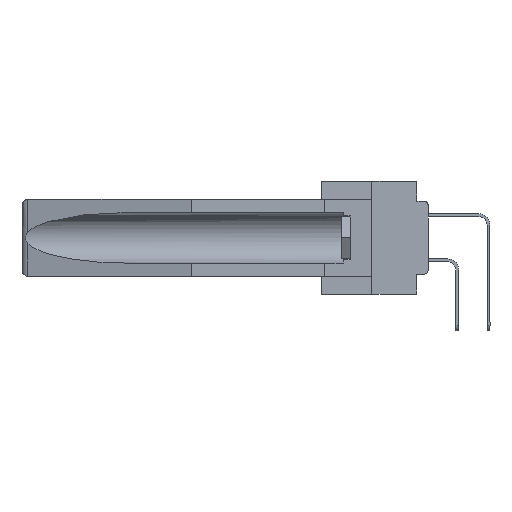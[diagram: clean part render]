
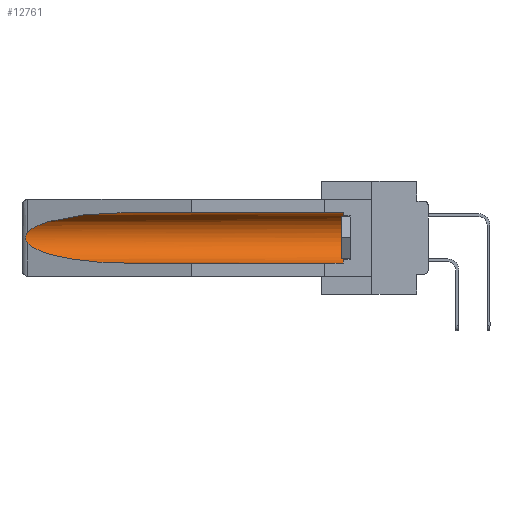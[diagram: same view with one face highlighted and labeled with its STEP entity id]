
A CAD part, left-side view. The second image highlights one B-rep face of the part: STEP entity #12761.
In plain terms, the highlighted cylindrical face has radius 2.857 mm (diameter 5.715 mm), a partial arc.
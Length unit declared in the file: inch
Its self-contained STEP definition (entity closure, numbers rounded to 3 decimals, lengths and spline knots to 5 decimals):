
#741 = DIRECTION ( 'NONE',  ( 0., -1., 0. ) ) ;
#1095 = VERTEX_POINT ( 'NONE', #1734 ) ;
#1589 = CARTESIAN_POINT ( 'NONE',  ( 0.26654, 1.53092, -0.15636 ) ) ;
#1707 =( BOUNDED_CURVE ( )  B_SPLINE_CURVE ( 3, ( #26544, #2659, #31917, #33365 ),
 .UNSPECIFIED., .F., .T. ) 
 B_SPLINE_CURVE_WITH_KNOTS ( ( 4, 4 ),
 ( 0.1948, 1.5708 ),
 .UNSPECIFIED. ) 
 CURVE ( )  GEOMETRIC_REPRESENTATION_ITEM ( )  RATIONAL_B_SPLINE_CURVE ( ( 1., 0.848, 0.848, 1. ) ) 
 REPRESENTATION_ITEM ( '' )  );
#1734 = CARTESIAN_POINT ( 'NONE',  ( 0.155, 0.126, -0.284 ) ) ;
#1753 = CARTESIAN_POINT ( 'NONE',  ( 0.155, 1.07973, -0.059 ) ) ;
#2185 = DIRECTION ( 'NONE',  ( 0., 1., 0. ) ) ;
#2433 = EDGE_CURVE ( 'NONE', #29137, #6163, #12590, .T. ) ;
#2659 = CARTESIAN_POINT ( 'NONE',  ( 0.25451, 1.48313, -0.24835 ) ) ;
#4751 = B_SPLINE_CURVE_WITH_KNOTS ( 'NONE', 3,
 ( #6805, #23032, #1589, #31147, #17606, #23197, #30980, #7320, #12388, #20214 ),
 .UNSPECIFIED., .F., .F.,
 ( 4, 2, 2, 2, 4 ),
 ( 0., 0.00029, 0.00058, 0.00087, 0.00117 ),
 .UNSPECIFIED. ) ;
#4790 = CYLINDRICAL_SURFACE ( 'NONE', #17360, 0.1125 ) ;
#5153 = EDGE_CURVE ( 'NONE', #28629, #29137, #23954, .T. ) ;
#5501 = ORIENTED_EDGE ( 'NONE', *, *, #9242, .T. ) ;
#6163 = VERTEX_POINT ( 'NONE', #24202 ) ;
#6591 = CARTESIAN_POINT ( 'NONE',  ( 0.155, -0.30754, -0.284 ) ) ;
#6805 = CARTESIAN_POINT ( 'NONE',  ( 0.26537, 1.52718, -0.14972 ) ) ;
#7320 = CARTESIAN_POINT ( 'NONE',  ( 0.26655, 1.53094, -0.18657 ) ) ;
#8758 = CARTESIAN_POINT ( 'NONE',  ( 0.26537, 1.52718, -0.19328 ) ) ;
#9242 = EDGE_CURVE ( 'NONE', #1095, #28629, #21501, .T. ) ;
#9428 = CARTESIAN_POINT ( 'NONE',  ( 0.26537, 1.52718, -0.14972 ) ) ;
#10366 = CARTESIAN_POINT ( 'NONE',  ( 0.155, -0.30754, -0.059 ) ) ;
#11535 = EDGE_CURVE ( 'NONE', #18109, #17452, #1707, .T. ) ;
#11882 = CARTESIAN_POINT ( 'NONE',  ( 0.21114, 1.30732, -0.059 ) ) ;
#12384 = CARTESIAN_POINT ( 'NONE',  ( 0.25451, 1.48313, -0.09465 ) ) ;
#12388 = CARTESIAN_POINT ( 'NONE',  ( 0.26597, 1.5296, -0.19026 ) ) ;
#12590 =( BOUNDED_CURVE ( )  B_SPLINE_CURVE ( 3, ( #1753, #11882, #12384, #9428 ),
 .UNSPECIFIED., .F., .T. ) 
 B_SPLINE_CURVE_WITH_KNOTS ( ( 4, 4 ),
 ( 4.71239, 6.08839 ),
 .UNSPECIFIED. ) 
 CURVE ( )  GEOMETRIC_REPRESENTATION_ITEM ( )  RATIONAL_B_SPLINE_CURVE ( ( 1., 0.848, 0.848, 1. ) ) 
 REPRESENTATION_ITEM ( '' )  );
#12638 = CARTESIAN_POINT ( 'NONE',  ( 0.155, 1.07973, -0.284 ) ) ;
#12761 = ADVANCED_FACE ( 'NONE', ( #30919 ), #4790, .F. ) ;
#12999 = DIRECTION ( 'NONE',  ( 0., 0., 1. ) ) ;
#14518 = CARTESIAN_POINT ( 'NONE',  ( 0.155, 0.126, -0.059 ) ) ;
#15182 = ORIENTED_EDGE ( 'NONE', *, *, #26651, .T. ) ;
#17360 = AXIS2_PLACEMENT_3D ( 'NONE', #28176, #2185, #12999 ) ;
#17452 = VERTEX_POINT ( 'NONE', #12638 ) ;
#17564 = DIRECTION ( 'NONE',  ( 0., 1., 0. ) ) ;
#17606 = CARTESIAN_POINT ( 'NONE',  ( 0.2675, 1.53308, -0.16763 ) ) ;
#17778 = ORIENTED_EDGE ( 'NONE', *, *, #32918, .F. ) ;
#18109 = VERTEX_POINT ( 'NONE', #8758 ) ;
#19148 = ORIENTED_EDGE ( 'NONE', *, *, #11535, .T. ) ;
#19695 = DIRECTION ( 'NONE',  ( 0., 0., 1. ) ) ;
#20214 = CARTESIAN_POINT ( 'NONE',  ( 0.26537, 1.52718, -0.19328 ) ) ;
#20800 = DIRECTION ( 'NONE',  ( 0., 1., 0. ) ) ;
#21501 = CIRCLE ( 'NONE', #33087, 0.1125 ) ;
#22136 = CARTESIAN_POINT ( 'NONE',  ( 0.155, 0.126, -0.1715 ) ) ;
#22277 = CARTESIAN_POINT ( 'NONE',  ( 0.155, 1.07973, -0.059 ) ) ;
#23031 = EDGE_LOOP ( 'NONE', ( #29703, #15182, #19148, #17778, #5501, #27229 ) ) ;
#23032 = CARTESIAN_POINT ( 'NONE',  ( 0.26597, 1.52961, -0.15275 ) ) ;
#23197 = CARTESIAN_POINT ( 'NONE',  ( 0.2675, 1.53308, -0.17534 ) ) ;
#23954 = LINE ( 'NONE', #10366, #32897 ) ;
#24202 = CARTESIAN_POINT ( 'NONE',  ( 0.26537, 1.52718, -0.14972 ) ) ;
#26544 = CARTESIAN_POINT ( 'NONE',  ( 0.26537, 1.52718, -0.19328 ) ) ;
#26651 = EDGE_CURVE ( 'NONE', #6163, #18109, #4751, .T. ) ;
#27229 = ORIENTED_EDGE ( 'NONE', *, *, #5153, .T. ) ;
#27854 = LINE ( 'NONE', #6591, #30821 ) ;
#28176 = CARTESIAN_POINT ( 'NONE',  ( 0.155, -0.30754, -0.1715 ) ) ;
#28629 = VERTEX_POINT ( 'NONE', #14518 ) ;
#29137 = VERTEX_POINT ( 'NONE', #22277 ) ;
#29703 = ORIENTED_EDGE ( 'NONE', *, *, #2433, .T. ) ;
#30821 = VECTOR ( 'NONE', #17564, 39.37008 ) ;
#30919 = FACE_OUTER_BOUND ( 'NONE', #23031, .T. ) ;
#30980 = CARTESIAN_POINT ( 'NONE',  ( 0.2673, 1.53269, -0.17917 ) ) ;
#31147 = CARTESIAN_POINT ( 'NONE',  ( 0.2673, 1.5327, -0.16383 ) ) ;
#31917 = CARTESIAN_POINT ( 'NONE',  ( 0.21114, 1.30732, -0.284 ) ) ;
#32897 = VECTOR ( 'NONE', #20800, 39.37008 ) ;
#32918 = EDGE_CURVE ( 'NONE', #1095, #17452, #27854, .T. ) ;
#33087 = AXIS2_PLACEMENT_3D ( 'NONE', #22136, #741, #19695 ) ;
#33365 = CARTESIAN_POINT ( 'NONE',  ( 0.155, 1.07973, -0.284 ) ) ;
